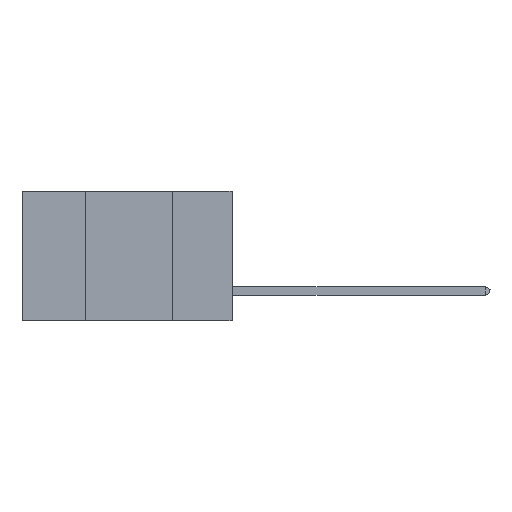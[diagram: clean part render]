
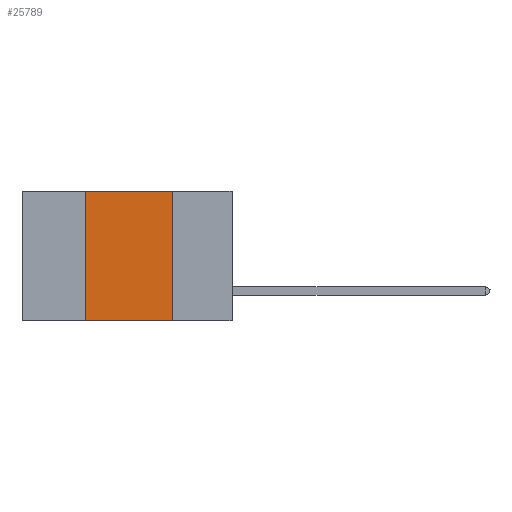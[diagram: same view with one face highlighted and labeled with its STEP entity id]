
A CAD part, left-side view. The second image highlights one B-rep face of the part: STEP entity #25789.
In plain terms, the highlighted planar face has unit normal (-1, 0, 0).
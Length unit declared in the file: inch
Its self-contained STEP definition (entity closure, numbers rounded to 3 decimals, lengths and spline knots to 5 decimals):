
#739 = LINE ( 'NONE', #31991, #7389 ) ;
#1845 = DIRECTION ( 'NONE',  ( 0., 0., -1. ) ) ;
#3686 = DIRECTION ( 'NONE',  ( 0., 0., 1. ) ) ;
#3811 = EDGE_CURVE ( 'NONE', #22549, #21614, #26077, .T. ) ;
#7389 = VECTOR ( 'NONE', #1845, 39.37008 ) ;
#7574 = PLANE ( 'NONE',  #29156 ) ;
#7585 = EDGE_CURVE ( 'NONE', #33067, #22549, #37095, .T. ) ;
#10061 = CARTESIAN_POINT ( 'NONE',  ( 0., 0.42, 0. ) ) ;
#10353 = ORIENTED_EDGE ( 'NONE', *, *, #7585, .F. ) ;
#10863 = DIRECTION ( 'NONE',  ( 0., 0., -1. ) ) ;
#11459 = CARTESIAN_POINT ( 'NONE',  ( 0., 0.17, 0. ) ) ;
#16133 = VECTOR ( 'NONE', #26048, 39.37008 ) ;
#21389 = ORIENTED_EDGE ( 'NONE', *, *, #3811, .F. ) ;
#21614 = VERTEX_POINT ( 'NONE', #11459 ) ;
#22023 = DIRECTION ( 'NONE',  ( 0., -1., 0. ) ) ;
#22289 = CARTESIAN_POINT ( 'NONE',  ( 0., 0.17, -0.37 ) ) ;
#22372 = EDGE_CURVE ( 'NONE', #33067, #27083, #31691, .T. ) ;
#22549 = VERTEX_POINT ( 'NONE', #10061 ) ;
#22933 = CARTESIAN_POINT ( 'NONE',  ( 0., 0.6, 0. ) ) ;
#23414 = FACE_OUTER_BOUND ( 'NONE', #28473, .T. ) ;
#23997 = EDGE_CURVE ( 'NONE', #21614, #27083, #739, .T. ) ;
#24722 = ORIENTED_EDGE ( 'NONE', *, *, #23997, .F. ) ;
#25789 = ADVANCED_FACE ( 'NONE', ( #23414 ), #7574, .F. ) ;
#26048 = DIRECTION ( 'NONE',  ( 0., -1., 0. ) ) ;
#26077 = LINE ( 'NONE', #32230, #16133 ) ;
#26238 = ORIENTED_EDGE ( 'NONE', *, *, #22372, .T. ) ;
#27083 = VERTEX_POINT ( 'NONE', #22289 ) ;
#27196 = VECTOR ( 'NONE', #3686, 39.37008 ) ;
#28473 = EDGE_LOOP ( 'NONE', ( #24722, #21389, #10353, #26238 ) ) ;
#29156 = AXIS2_PLACEMENT_3D ( 'NONE', #22933, #38890, #10863 ) ;
#30927 = CARTESIAN_POINT ( 'NONE',  ( 0., 0.42, 0. ) ) ;
#31691 = LINE ( 'NONE', #37437, #38793 ) ;
#31991 = CARTESIAN_POINT ( 'NONE',  ( 0., 0.17, 0. ) ) ;
#32230 = CARTESIAN_POINT ( 'NONE',  ( 0., 0.6, 0. ) ) ;
#33067 = VERTEX_POINT ( 'NONE', #34338 ) ;
#34338 = CARTESIAN_POINT ( 'NONE',  ( 0., 0.42, -0.37 ) ) ;
#37095 = LINE ( 'NONE', #30927, #27196 ) ;
#37437 = CARTESIAN_POINT ( 'NONE',  ( 0., 0.6, -0.37 ) ) ;
#38793 = VECTOR ( 'NONE', #22023, 39.37008 ) ;
#38890 = DIRECTION ( 'NONE',  ( 1., 0., 0. ) ) ;
